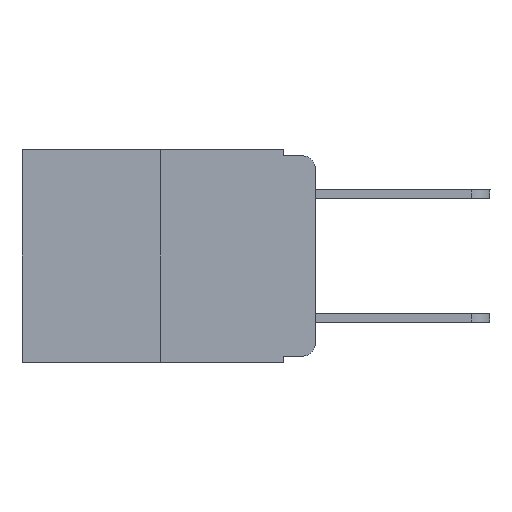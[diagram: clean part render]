
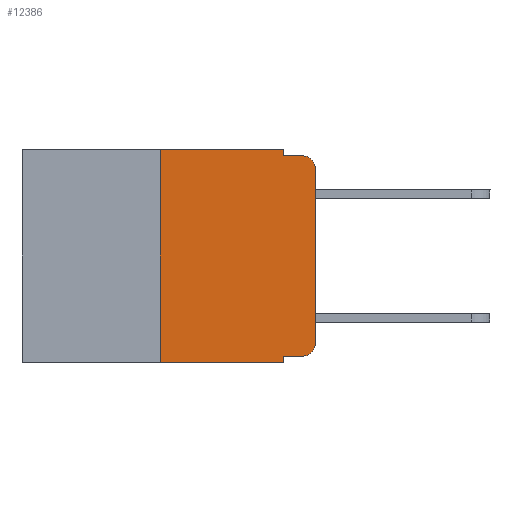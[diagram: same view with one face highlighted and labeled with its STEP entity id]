
A CAD part, left-side view. The second image highlights one B-rep face of the part: STEP entity #12386.
In plain terms, the highlighted planar face has unit normal (-1, 0, 0).
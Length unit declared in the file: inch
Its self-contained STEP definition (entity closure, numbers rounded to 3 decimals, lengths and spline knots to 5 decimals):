
#26 = CARTESIAN_POINT ( 'NONE',  ( 0., 0.051, -0.343 ) ) ;
#51 = LINE ( 'NONE', #4294, #17020 ) ;
#60 = CARTESIAN_POINT ( 'NONE',  ( 0., 0.02, -0.03 ) ) ;
#133 = VERTEX_POINT ( 'NONE', #8727 ) ;
#615 = EDGE_CURVE ( 'NONE', #15026, #5372, #3279, .T. ) ;
#650 = FACE_OUTER_BOUND ( 'NONE', #9107, .T. ) ;
#714 = ORIENTED_EDGE ( 'NONE', *, *, #615, .F. ) ;
#748 = VECTOR ( 'NONE', #13368, 39.37008 ) ;
#929 = LINE ( 'NONE', #6190, #15380 ) ;
#1069 = CARTESIAN_POINT ( 'NONE',  ( 0., 0.02, -0.333 ) ) ;
#1170 = VERTEX_POINT ( 'NONE', #7780 ) ;
#1273 = ORIENTED_EDGE ( 'NONE', *, *, #8272, .T. ) ;
#1647 = DIRECTION ( 'NONE',  ( 0., -1., 0. ) ) ;
#1700 = CARTESIAN_POINT ( 'NONE',  ( 0., 0., -0.03 ) ) ;
#1804 = AXIS2_PLACEMENT_3D ( 'NONE', #60, #11687, #6358 ) ;
#1818 = EDGE_CURVE ( 'NONE', #1170, #13402, #2424, .T. ) ;
#1952 = EDGE_CURVE ( 'NONE', #133, #5475, #15991, .T. ) ;
#1984 = DIRECTION ( 'NONE',  ( 0., -1., 0. ) ) ;
#1987 = ORIENTED_EDGE ( 'NONE', *, *, #1818, .T. ) ;
#2424 = LINE ( 'NONE', #12685, #7130 ) ;
#2539 = VERTEX_POINT ( 'NONE', #15342 ) ;
#2704 = ORIENTED_EDGE ( 'NONE', *, *, #16053, .F. ) ;
#2738 = VECTOR ( 'NONE', #9406, 39.37008 ) ;
#2867 = LINE ( 'NONE', #9155, #748 ) ;
#2962 = CARTESIAN_POINT ( 'NONE',  ( 0., 0.473, 0. ) ) ;
#3279 = LINE ( 'NONE', #8530, #6945 ) ;
#3855 = DIRECTION ( 'NONE',  ( 0., 0., -1. ) ) ;
#4164 = CARTESIAN_POINT ( 'NONE',  ( 0., 0.473, 0. ) ) ;
#4294 = CARTESIAN_POINT ( 'NONE',  ( 0., 0.25, 0. ) ) ;
#4385 = ORIENTED_EDGE ( 'NONE', *, *, #1952, .F. ) ;
#4575 = DIRECTION ( 'NONE',  ( 0., 0., -1. ) ) ;
#5327 = CARTESIAN_POINT ( 'NONE',  ( 0., 0.02, -0.01 ) ) ;
#5372 = VERTEX_POINT ( 'NONE', #5327 ) ;
#5475 = VERTEX_POINT ( 'NONE', #6537 ) ;
#6190 = CARTESIAN_POINT ( 'NONE',  ( 0., 0.051, 0. ) ) ;
#6343 = EDGE_CURVE ( 'NONE', #16277, #7697, #13195, .T. ) ;
#6358 = DIRECTION ( 'NONE',  ( 0., 0., -1. ) ) ;
#6537 = CARTESIAN_POINT ( 'NONE',  ( 0., 0.051, 0. ) ) ;
#6945 = VECTOR ( 'NONE', #1984, 39.37008 ) ;
#7044 = ORIENTED_EDGE ( 'NONE', *, *, #10951, .F. ) ;
#7130 = VECTOR ( 'NONE', #7769, 39.37008 ) ;
#7565 = VERTEX_POINT ( 'NONE', #1069 ) ;
#7697 = VERTEX_POINT ( 'NONE', #26 ) ;
#7769 = DIRECTION ( 'NONE',  ( 0., 0., 1. ) ) ;
#7780 = CARTESIAN_POINT ( 'NONE',  ( 0., 0., -0.313 ) ) ;
#7982 = DIRECTION ( 'NONE',  ( 0., 0., 1. ) ) ;
#8088 = ORIENTED_EDGE ( 'NONE', *, *, #14820, .F. ) ;
#8272 = EDGE_CURVE ( 'NONE', #7565, #1170, #14675, .T. ) ;
#8396 = CARTESIAN_POINT ( 'NONE',  ( 0., 0.051, 0. ) ) ;
#8530 = CARTESIAN_POINT ( 'NONE',  ( 0., 0.051, -0.01 ) ) ;
#8727 = CARTESIAN_POINT ( 'NONE',  ( 0., 0.25, 0. ) ) ;
#9107 = EDGE_LOOP ( 'NONE', ( #1987, #10298, #714, #2704, #4385, #8088, #14718, #7044, #9706, #1273 ) ) ;
#9155 = CARTESIAN_POINT ( 'NONE',  ( 0., 0.051, -0.333 ) ) ;
#9406 = DIRECTION ( 'NONE',  ( 0., -1., 0. ) ) ;
#9510 = CIRCLE ( 'NONE', #1804, 0.02 ) ;
#9683 = LINE ( 'NONE', #8396, #16028 ) ;
#9706 = ORIENTED_EDGE ( 'NONE', *, *, #13952, .T. ) ;
#9900 = DIRECTION ( 'NONE',  ( -1., 0., 0. ) ) ;
#10298 = ORIENTED_EDGE ( 'NONE', *, *, #11945, .T. ) ;
#10384 = DIRECTION ( 'NONE',  ( 1., 0., 0. ) ) ;
#10795 = AXIS2_PLACEMENT_3D ( 'NONE', #11092, #9900, #4575 ) ;
#10951 = EDGE_CURVE ( 'NONE', #2539, #7697, #9683, .T. ) ;
#11045 = DIRECTION ( 'NONE',  ( 0., 0., -1. ) ) ;
#11092 = CARTESIAN_POINT ( 'NONE',  ( 0., 0.02, -0.313 ) ) ;
#11428 = DIRECTION ( 'NONE',  ( 0., 0., -1. ) ) ;
#11687 = DIRECTION ( 'NONE',  ( -1., 0., 0. ) ) ;
#11945 = EDGE_CURVE ( 'NONE', #13402, #5372, #9510, .T. ) ;
#12386 = ADVANCED_FACE ( 'NONE', ( #650 ), #15590, .F. ) ;
#12685 = CARTESIAN_POINT ( 'NONE',  ( 0., 0., 0. ) ) ;
#13195 = LINE ( 'NONE', #14595, #13231 ) ;
#13231 = VECTOR ( 'NONE', #1647, 39.37008 ) ;
#13368 = DIRECTION ( 'NONE',  ( 0., -1., 0. ) ) ;
#13402 = VERTEX_POINT ( 'NONE', #1700 ) ;
#13853 = CARTESIAN_POINT ( 'NONE',  ( 0., 0.25, -0.343 ) ) ;
#13952 = EDGE_CURVE ( 'NONE', #2539, #7565, #2867, .T. ) ;
#14595 = CARTESIAN_POINT ( 'NONE',  ( 0., 0.473, -0.343 ) ) ;
#14675 = CIRCLE ( 'NONE', #10795, 0.02 ) ;
#14718 = ORIENTED_EDGE ( 'NONE', *, *, #6343, .T. ) ;
#14773 = AXIS2_PLACEMENT_3D ( 'NONE', #2962, #10384, #3855 ) ;
#14820 = EDGE_CURVE ( 'NONE', #16277, #133, #51, .T. ) ;
#15026 = VERTEX_POINT ( 'NONE', #16538 ) ;
#15342 = CARTESIAN_POINT ( 'NONE',  ( 0., 0.051, -0.333 ) ) ;
#15380 = VECTOR ( 'NONE', #11428, 39.37008 ) ;
#15590 = PLANE ( 'NONE',  #14773 ) ;
#15991 = LINE ( 'NONE', #4164, #2738 ) ;
#16028 = VECTOR ( 'NONE', #11045, 39.37008 ) ;
#16053 = EDGE_CURVE ( 'NONE', #5475, #15026, #929, .T. ) ;
#16277 = VERTEX_POINT ( 'NONE', #13853 ) ;
#16538 = CARTESIAN_POINT ( 'NONE',  ( 0., 0.051, -0.01 ) ) ;
#17020 = VECTOR ( 'NONE', #7982, 39.37008 ) ;
